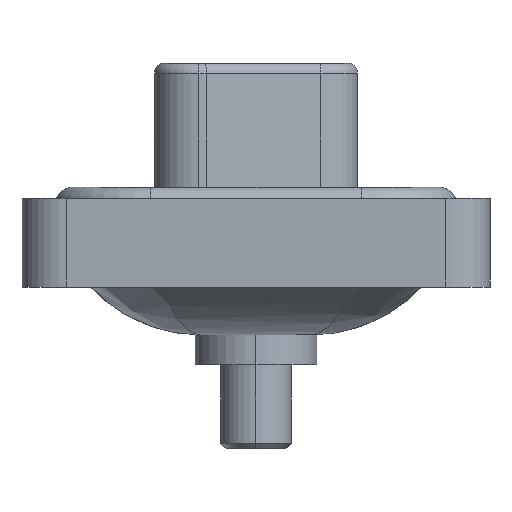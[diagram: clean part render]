
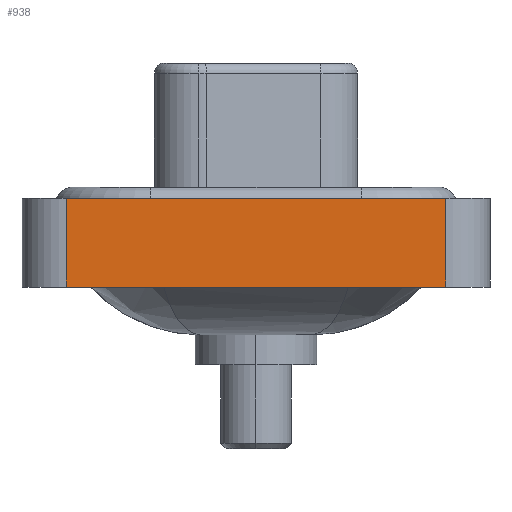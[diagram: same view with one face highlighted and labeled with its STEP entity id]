
A CAD part, left-side view. The second image highlights one B-rep face of the part: STEP entity #938.
In plain terms, the highlighted planar face has unit normal (-1, 0, 0).
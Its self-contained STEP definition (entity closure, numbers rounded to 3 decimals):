
#471 = EDGE_CURVE ( 'NONE', #11990, #8681, #11050, .T. ) ;
#728 = CARTESIAN_POINT ( 'NONE',  ( -7.25, -8.55, -3.6 ) ) ;
#938 = ADVANCED_FACE ( 'NONE', ( #14521 ), #6383, .T. ) ;
#1138 = CARTESIAN_POINT ( 'NONE',  ( -7.25, 8.55, 0.4 ) ) ;
#1214 = AXIS2_PLACEMENT_3D ( 'NONE', #1843, #9807, #14436 ) ;
#1484 = EDGE_CURVE ( 'NONE', #11990, #6828, #4869, .T. ) ;
#1554 = DIRECTION ( 'NONE',  ( 0., 0., 1. ) ) ;
#1843 = CARTESIAN_POINT ( 'NONE',  ( -7.25, -8.55, -3.6 ) ) ;
#2616 = CARTESIAN_POINT ( 'NONE',  ( -7.25, 8.55, -3.6 ) ) ;
#3269 = CARTESIAN_POINT ( 'NONE',  ( -7.25, -8.55, -3.6 ) ) ;
#3638 = EDGE_CURVE ( 'NONE', #6828, #10116, #4549, .T. ) ;
#4549 = LINE ( 'NONE', #12517, #14805 ) ;
#4869 = LINE ( 'NONE', #10663, #14555 ) ;
#5307 = EDGE_LOOP ( 'NONE', ( #12325, #6510, #7129, #8827 ) ) ;
#5526 = DIRECTION ( 'NONE',  ( 0., -1., 0. ) ) ;
#6383 = PLANE ( 'NONE',  #1214 ) ;
#6510 = ORIENTED_EDGE ( 'NONE', *, *, #3638, .F. ) ;
#6828 = VERTEX_POINT ( 'NONE', #1138 ) ;
#7129 = ORIENTED_EDGE ( 'NONE', *, *, #1484, .F. ) ;
#8134 = VECTOR ( 'NONE', #14844, 1000. ) ;
#8681 = VERTEX_POINT ( 'NONE', #3269 ) ;
#8827 = ORIENTED_EDGE ( 'NONE', *, *, #471, .T. ) ;
#9357 = VECTOR ( 'NONE', #14753, 1000. ) ;
#9807 = DIRECTION ( 'NONE',  ( -1., 0., 0. ) ) ;
#9851 = EDGE_CURVE ( 'NONE', #8681, #10116, #12480, .T. ) ;
#10116 = VERTEX_POINT ( 'NONE', #11953 ) ;
#10211 = CARTESIAN_POINT ( 'NONE',  ( -7.25, -8.55, -3.6 ) ) ;
#10663 = CARTESIAN_POINT ( 'NONE',  ( -7.25, 8.55, -3.6 ) ) ;
#11050 = LINE ( 'NONE', #728, #9357 ) ;
#11953 = CARTESIAN_POINT ( 'NONE',  ( -7.25, -8.55, 0.4 ) ) ;
#11990 = VERTEX_POINT ( 'NONE', #2616 ) ;
#12325 = ORIENTED_EDGE ( 'NONE', *, *, #9851, .T. ) ;
#12480 = LINE ( 'NONE', #10211, #8134 ) ;
#12517 = CARTESIAN_POINT ( 'NONE',  ( -7.25, -8.55, 0.4 ) ) ;
#14436 = DIRECTION ( 'NONE',  ( 0., 0., 1. ) ) ;
#14521 = FACE_OUTER_BOUND ( 'NONE', #5307, .T. ) ;
#14555 = VECTOR ( 'NONE', #1554, 1000. ) ;
#14753 = DIRECTION ( 'NONE',  ( 0., -1., 0. ) ) ;
#14805 = VECTOR ( 'NONE', #5526, 1000. ) ;
#14844 = DIRECTION ( 'NONE',  ( 0., 0., 1. ) ) ;
